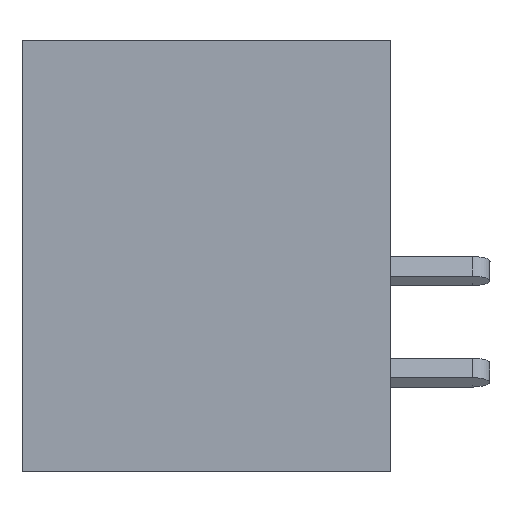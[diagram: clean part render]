
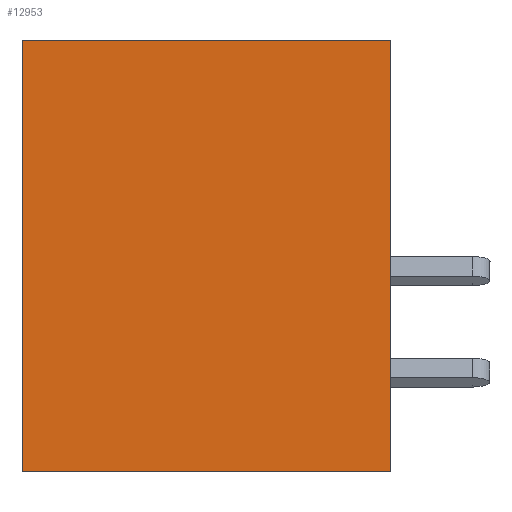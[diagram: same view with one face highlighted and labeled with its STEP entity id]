
A CAD part, left-side view. The second image highlights one B-rep face of the part: STEP entity #12953.
In plain terms, the highlighted planar face has unit normal (-1, 0, 0).
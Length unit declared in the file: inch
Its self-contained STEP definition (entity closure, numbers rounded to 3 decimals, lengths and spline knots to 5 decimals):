
#1152 = CARTESIAN_POINT ( 'NONE',  ( 0., 0., 0. ) ) ;
#2893 = VECTOR ( 'NONE', #5693, 39.37008 ) ;
#3603 = LINE ( 'NONE', #1152, #2893 ) ;
#3768 = DIRECTION ( 'NONE',  ( 0., -1., 0. ) ) ;
#4140 = DIRECTION ( 'NONE',  ( 1., 0., 0. ) ) ;
#4799 = VECTOR ( 'NONE', #3768, 39.37008 ) ;
#5284 = VECTOR ( 'NONE', #10504, 39.37008 ) ;
#5693 = DIRECTION ( 'NONE',  ( 0., 0., 1. ) ) ;
#6908 = EDGE_LOOP ( 'NONE', ( #11332, #15844, #12938, #15357 ) ) ;
#7046 = CARTESIAN_POINT ( 'NONE',  ( 0., 0., -0.531 ) ) ;
#7595 = CARTESIAN_POINT ( 'NONE',  ( 0., 0.453, 0. ) ) ;
#8559 = LINE ( 'NONE', #7595, #5284 ) ;
#9185 = CARTESIAN_POINT ( 'NONE',  ( 0., 0.453, 0. ) ) ;
#9832 = VERTEX_POINT ( 'NONE', #18154 ) ;
#10504 = DIRECTION ( 'NONE',  ( 0., -1., 0. ) ) ;
#11332 = ORIENTED_EDGE ( 'NONE', *, *, #13118, .T. ) ;
#11568 = DIRECTION ( 'NONE',  ( 0., 0., 1. ) ) ;
#11734 = EDGE_CURVE ( 'NONE', #16051, #13021, #18144, .T. ) ;
#12231 = EDGE_CURVE ( 'NONE', #13021, #9832, #8559, .T. ) ;
#12378 = EDGE_CURVE ( 'NONE', #16051, #16237, #17660, .T. ) ;
#12749 = CARTESIAN_POINT ( 'NONE',  ( 0., 0.453, -0.531 ) ) ;
#12938 = ORIENTED_EDGE ( 'NONE', *, *, #11734, .F. ) ;
#12953 = ADVANCED_FACE ( 'NONE', ( #14559 ), #15876, .F. ) ;
#13021 = VERTEX_POINT ( 'NONE', #9185 ) ;
#13118 = EDGE_CURVE ( 'NONE', #16237, #9832, #3603, .T. ) ;
#14559 = FACE_OUTER_BOUND ( 'NONE', #6908, .T. ) ;
#15103 = AXIS2_PLACEMENT_3D ( 'NONE', #18888, #4140, #17527 ) ;
#15357 = ORIENTED_EDGE ( 'NONE', *, *, #12378, .T. ) ;
#15844 = ORIENTED_EDGE ( 'NONE', *, *, #12231, .F. ) ;
#15876 = PLANE ( 'NONE',  #15103 ) ;
#16051 = VERTEX_POINT ( 'NONE', #19086 ) ;
#16237 = VERTEX_POINT ( 'NONE', #7046 ) ;
#16264 = CARTESIAN_POINT ( 'NONE',  ( 0., 0.453, 0. ) ) ;
#17527 = DIRECTION ( 'NONE',  ( 0., 0., -1. ) ) ;
#17660 = LINE ( 'NONE', #12749, #4799 ) ;
#17927 = VECTOR ( 'NONE', #11568, 39.37008 ) ;
#18144 = LINE ( 'NONE', #16264, #17927 ) ;
#18154 = CARTESIAN_POINT ( 'NONE',  ( 0., 0., 0. ) ) ;
#18888 = CARTESIAN_POINT ( 'NONE',  ( 0., 0.453, 0. ) ) ;
#19086 = CARTESIAN_POINT ( 'NONE',  ( 0., 0.453, -0.531 ) ) ;
